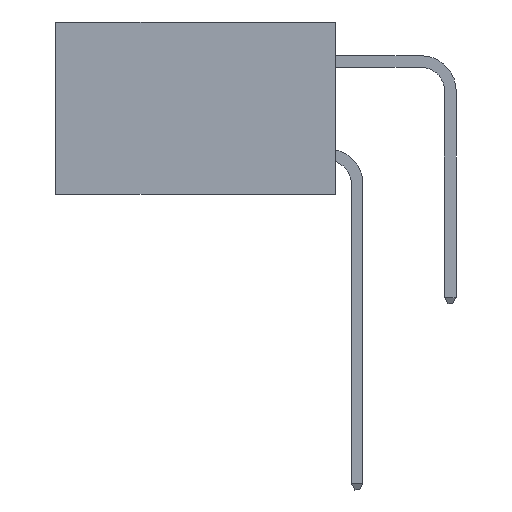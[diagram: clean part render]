
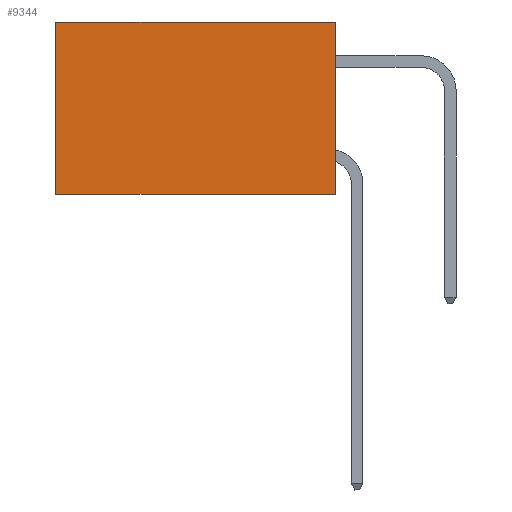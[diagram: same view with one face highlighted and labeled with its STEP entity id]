
A CAD part, left-side view. The second image highlights one B-rep face of the part: STEP entity #9344.
In plain terms, the highlighted planar face has unit normal (-1, 0, 0).
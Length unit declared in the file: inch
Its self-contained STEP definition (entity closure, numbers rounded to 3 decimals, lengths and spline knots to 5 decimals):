
#1 = DIRECTION ( 'NONE',  ( 0., 1., 0. ) ) ;
#188 = CARTESIAN_POINT ( 'NONE',  ( 0.2875, 0., 0. ) ) ;
#432 = ORIENTED_EDGE ( 'NONE', *, *, #17141, .F. ) ;
#611 = CARTESIAN_POINT ( 'NONE',  ( 0.2875, 0., -0.37 ) ) ;
#653 = CARTESIAN_POINT ( 'NONE',  ( 0.2875, 0., 0. ) ) ;
#1371 = VERTEX_POINT ( 'NONE', #12865 ) ;
#1613 = EDGE_LOOP ( 'NONE', ( #7766, #432, #18791, #17522 ) ) ;
#2397 = VECTOR ( 'NONE', #15839, 39.37008 ) ;
#3734 = LINE ( 'NONE', #8345, #6751 ) ;
#6273 = VECTOR ( 'NONE', #16245, 39.37008 ) ;
#6280 = AXIS2_PLACEMENT_3D ( 'NONE', #11418, #8417, #15843 ) ;
#6751 = VECTOR ( 'NONE', #6998, 39.37008 ) ;
#6998 = DIRECTION ( 'NONE',  ( 0., 1., 0. ) ) ;
#7415 = EDGE_CURVE ( 'NONE', #8072, #1371, #16935, .T. ) ;
#7470 = LINE ( 'NONE', #19393, #6273 ) ;
#7766 = ORIENTED_EDGE ( 'NONE', *, *, #8677, .T. ) ;
#8072 = VERTEX_POINT ( 'NONE', #14348 ) ;
#8345 = CARTESIAN_POINT ( 'NONE',  ( 0.2875, 0., -0.37 ) ) ;
#8417 = DIRECTION ( 'NONE',  ( 1., 0., 0. ) ) ;
#8677 = EDGE_CURVE ( 'NONE', #1371, #11581, #7470, .T. ) ;
#9344 = ADVANCED_FACE ( 'NONE', ( #17779 ), #11281, .F. ) ;
#9879 = CARTESIAN_POINT ( 'NONE',  ( 0.2875, 0.6, -0.37 ) ) ;
#11281 = PLANE ( 'NONE',  #6280 ) ;
#11418 = CARTESIAN_POINT ( 'NONE',  ( 0.2875, 0., 0. ) ) ;
#11581 = VERTEX_POINT ( 'NONE', #9879 ) ;
#12865 = CARTESIAN_POINT ( 'NONE',  ( 0.2875, 0.6, 0. ) ) ;
#14348 = CARTESIAN_POINT ( 'NONE',  ( 0.2875, 0., 0. ) ) ;
#14932 = EDGE_CURVE ( 'NONE', #8072, #19003, #16684, .T. ) ;
#15537 = VECTOR ( 'NONE', #1, 39.37008 ) ;
#15839 = DIRECTION ( 'NONE',  ( 0., 0., -1. ) ) ;
#15843 = DIRECTION ( 'NONE',  ( 0., 0., -1. ) ) ;
#16245 = DIRECTION ( 'NONE',  ( 0., 0., -1. ) ) ;
#16684 = LINE ( 'NONE', #653, #2397 ) ;
#16935 = LINE ( 'NONE', #188, #15537 ) ;
#17141 = EDGE_CURVE ( 'NONE', #19003, #11581, #3734, .T. ) ;
#17522 = ORIENTED_EDGE ( 'NONE', *, *, #7415, .T. ) ;
#17779 = FACE_OUTER_BOUND ( 'NONE', #1613, .T. ) ;
#18791 = ORIENTED_EDGE ( 'NONE', *, *, #14932, .F. ) ;
#19003 = VERTEX_POINT ( 'NONE', #611 ) ;
#19393 = CARTESIAN_POINT ( 'NONE',  ( 0.2875, 0.6, 0. ) ) ;
